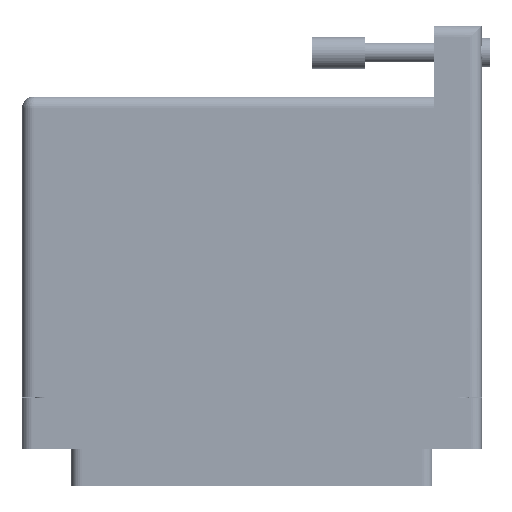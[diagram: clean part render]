
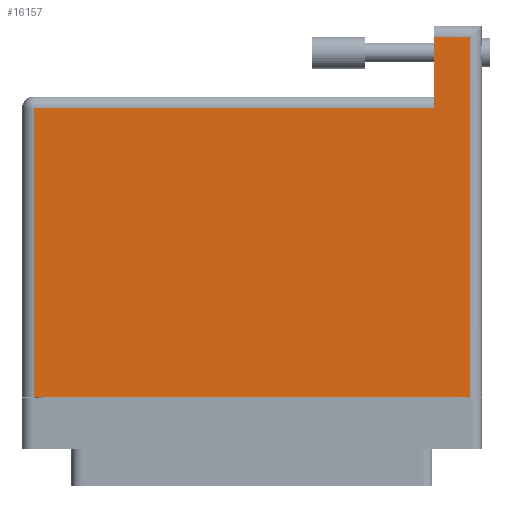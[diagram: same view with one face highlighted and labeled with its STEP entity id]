
A CAD part, front view. The second image highlights one B-rep face of the part: STEP entity #16157.
In plain terms, the highlighted face is planar.
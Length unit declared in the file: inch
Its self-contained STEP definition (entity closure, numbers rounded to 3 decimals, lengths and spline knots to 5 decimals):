
#3439 = EDGE_CURVE ( 'NONE', #19114, #63176, #26714, .T. ) ;
#3522 = CARTESIAN_POINT ( 'NONE',  ( -1.359, 1.675, 0.617 ) ) ;
#4444 = AXIS2_PLACEMENT_3D ( 'NONE', #3522, #72113, #49478 ) ;
#4841 = EDGE_CURVE ( 'NONE', #34037, #52716, #71564, .T. ) ;
#5567 = CARTESIAN_POINT ( 'NONE',  ( -1.289, -0.1, 0.617 ) ) ;
#5848 = CARTESIAN_POINT ( 'NONE',  ( 1.079, 1.605, 0.617 ) ) ;
#6318 = VECTOR ( 'NONE', #33352, 39.37008 ) ;
#6346 = EDGE_CURVE ( 'NONE', #26822, #19114, #31185, .T. ) ;
#6576 = VECTOR ( 'NONE', #35712, 39.37008 ) ;
#9738 = EDGE_CURVE ( 'NONE', #52716, #26822, #67407, .T. ) ;
#11396 = CARTESIAN_POINT ( 'NONE',  ( -1.289, -0.1, 0.617 ) ) ;
#11530 = VERTEX_POINT ( 'NONE', #62770 ) ;
#13426 = DIRECTION ( 'NONE',  ( 1., 0., 0. ) ) ;
#16157 = ADVANCED_FACE ( 'NONE', ( #30826 ), #55208, .F. ) ;
#17936 = LINE ( 'NONE', #55713, #58813 ) ;
#18327 = CARTESIAN_POINT ( 'NONE',  ( 1.079, 2.025, 0.617 ) ) ;
#19114 = VERTEX_POINT ( 'NONE', #18327 ) ;
#21626 = DIRECTION ( 'NONE',  ( -1., 0., 0. ) ) ;
#24577 = VECTOR ( 'NONE', #38086, 39.37008 ) ;
#26714 = LINE ( 'NONE', #54713, #29320 ) ;
#26822 = VERTEX_POINT ( 'NONE', #37461 ) ;
#27029 = LINE ( 'NONE', #11396, #6576 ) ;
#27662 = ORIENTED_EDGE ( 'NONE', *, *, #68295, .T. ) ;
#29320 = VECTOR ( 'NONE', #31762, 39.37008 ) ;
#30826 = FACE_OUTER_BOUND ( 'NONE', #66818, .T. ) ;
#31185 = LINE ( 'NONE', #62252, #6318 ) ;
#31762 = DIRECTION ( 'NONE',  ( 0., -1., 0. ) ) ;
#33352 = DIRECTION ( 'NONE',  ( -1., 0., 0. ) ) ;
#34037 = VERTEX_POINT ( 'NONE', #5567 ) ;
#35524 = CARTESIAN_POINT ( 'NONE',  ( -1.359, -0.1, 0.617 ) ) ;
#35712 = DIRECTION ( 'NONE',  ( 0., -1., 0. ) ) ;
#37461 = CARTESIAN_POINT ( 'NONE',  ( 1.289, 2.025, 0.617 ) ) ;
#37605 = CARTESIAN_POINT ( 'NONE',  ( 1.289, 2.095, 0.617 ) ) ;
#37739 = VECTOR ( 'NONE', #13426, 39.37008 ) ;
#38071 = ORIENTED_EDGE ( 'NONE', *, *, #60020, .T. ) ;
#38086 = DIRECTION ( 'NONE',  ( 0., 1., 0. ) ) ;
#43922 = ORIENTED_EDGE ( 'NONE', *, *, #6346, .T. ) ;
#45194 = ORIENTED_EDGE ( 'NONE', *, *, #4841, .T. ) ;
#47744 = ORIENTED_EDGE ( 'NONE', *, *, #9738, .T. ) ;
#49478 = DIRECTION ( 'NONE',  ( -1., 0., 0. ) ) ;
#52716 = VERTEX_POINT ( 'NONE', #55631 ) ;
#54713 = CARTESIAN_POINT ( 'NONE',  ( 1.079, 2.095, 0.617 ) ) ;
#55208 = PLANE ( 'NONE',  #4444 ) ;
#55631 = CARTESIAN_POINT ( 'NONE',  ( 1.289, -0.1, 0.617 ) ) ;
#55713 = CARTESIAN_POINT ( 'NONE',  ( -1.359, 1.605, 0.617 ) ) ;
#58813 = VECTOR ( 'NONE', #21626, 39.37008 ) ;
#60020 = EDGE_CURVE ( 'NONE', #63176, #11530, #17936, .T. ) ;
#61275 = ORIENTED_EDGE ( 'NONE', *, *, #3439, .T. ) ;
#62252 = CARTESIAN_POINT ( 'NONE',  ( -1.359, 2.025, 0.617 ) ) ;
#62770 = CARTESIAN_POINT ( 'NONE',  ( -1.289, 1.605, 0.617 ) ) ;
#63176 = VERTEX_POINT ( 'NONE', #5848 ) ;
#66818 = EDGE_LOOP ( 'NONE', ( #38071, #27662, #45194, #47744, #43922, #61275 ) ) ;
#67407 = LINE ( 'NONE', #37605, #24577 ) ;
#68295 = EDGE_CURVE ( 'NONE', #11530, #34037, #27029, .T. ) ;
#71564 = LINE ( 'NONE', #35524, #37739 ) ;
#72113 = DIRECTION ( 'NONE',  ( 0., 0., -1. ) ) ;
